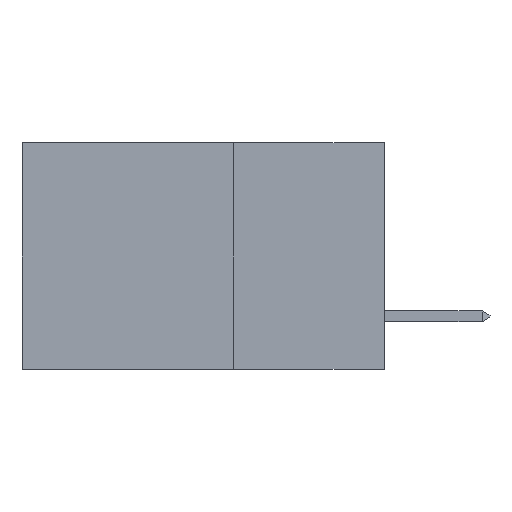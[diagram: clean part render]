
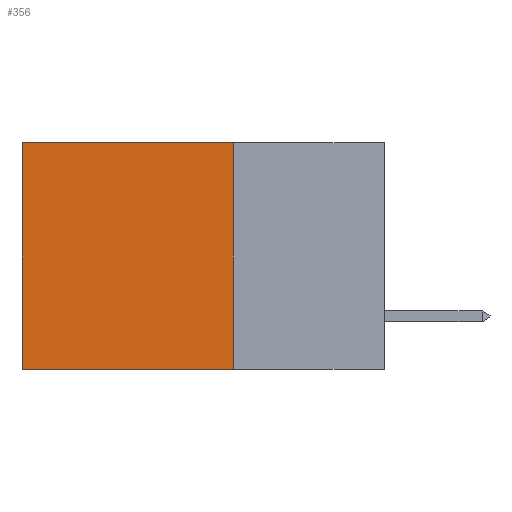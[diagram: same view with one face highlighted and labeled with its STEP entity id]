
A CAD part, left-side view. The second image highlights one B-rep face of the part: STEP entity #356.
In plain terms, the highlighted planar face has unit normal (-1, 0, 0).
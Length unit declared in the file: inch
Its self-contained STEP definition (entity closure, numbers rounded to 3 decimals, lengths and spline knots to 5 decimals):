
#85 = VECTOR ( 'NONE', #6011, 39.37008 ) ;
#267 = VECTOR ( 'NONE', #5289, 39.37008 ) ;
#356 = ADVANCED_FACE ( 'NONE', ( #3640 ), #1691, .F. ) ;
#379 = LINE ( 'NONE', #4666, #5383 ) ;
#416 = CARTESIAN_POINT ( 'NONE',  ( 0.2875, 0.6, -0.375 ) ) ;
#968 = VERTEX_POINT ( 'NONE', #416 ) ;
#1175 = CARTESIAN_POINT ( 'NONE',  ( 0.2875, 0.25, -0.375 ) ) ;
#1236 = CARTESIAN_POINT ( 'NONE',  ( 0.2875, 0.25, -0.375 ) ) ;
#1272 = ORIENTED_EDGE ( 'NONE', *, *, #5631, .F. ) ;
#1691 = PLANE ( 'NONE',  #5895 ) ;
#1702 = VECTOR ( 'NONE', #7063, 39.37008 ) ;
#2240 = VERTEX_POINT ( 'NONE', #5299 ) ;
#2464 = CARTESIAN_POINT ( 'NONE',  ( 0.2875, 0.25, 0. ) ) ;
#2891 = ORIENTED_EDGE ( 'NONE', *, *, #5147, .T. ) ;
#3093 = EDGE_LOOP ( 'NONE', ( #2891, #4474, #1272, #4085 ) ) ;
#3130 = CARTESIAN_POINT ( 'NONE',  ( 0.2875, 0.25, 0. ) ) ;
#3260 = LINE ( 'NONE', #5329, #85 ) ;
#3342 = LINE ( 'NONE', #4630, #267 ) ;
#3640 = FACE_OUTER_BOUND ( 'NONE', #3093, .T. ) ;
#3717 = LINE ( 'NONE', #2464, #1702 ) ;
#4085 = ORIENTED_EDGE ( 'NONE', *, *, #6724, .T. ) ;
#4312 = VERTEX_POINT ( 'NONE', #3130 ) ;
#4474 = ORIENTED_EDGE ( 'NONE', *, *, #6295, .F. ) ;
#4578 = DIRECTION ( 'NONE',  ( 0., 0., -1. ) ) ;
#4630 = CARTESIAN_POINT ( 'NONE',  ( 0.2875, 0.25, -0.375 ) ) ;
#4666 = CARTESIAN_POINT ( 'NONE',  ( 0.2875, 0.25, -0.375 ) ) ;
#4964 = DIRECTION ( 'NONE',  ( 0., 0., -1. ) ) ;
#5147 = EDGE_CURVE ( 'NONE', #2240, #968, #3260, .T. ) ;
#5289 = DIRECTION ( 'NONE',  ( 0., 1., 0. ) ) ;
#5299 = CARTESIAN_POINT ( 'NONE',  ( 0.2875, 0.6, 0. ) ) ;
#5329 = CARTESIAN_POINT ( 'NONE',  ( 0.2875, 0.6, -0.375 ) ) ;
#5383 = VECTOR ( 'NONE', #4578, 39.37008 ) ;
#5631 = EDGE_CURVE ( 'NONE', #4312, #7329, #379, .T. ) ;
#5895 = AXIS2_PLACEMENT_3D ( 'NONE', #1175, #6239, #4964 ) ;
#6011 = DIRECTION ( 'NONE',  ( 0., 0., -1. ) ) ;
#6239 = DIRECTION ( 'NONE',  ( 1., 0., 0. ) ) ;
#6295 = EDGE_CURVE ( 'NONE', #7329, #968, #3342, .T. ) ;
#6724 = EDGE_CURVE ( 'NONE', #4312, #2240, #3717, .T. ) ;
#7063 = DIRECTION ( 'NONE',  ( 0., 1., 0. ) ) ;
#7329 = VERTEX_POINT ( 'NONE', #1236 ) ;
